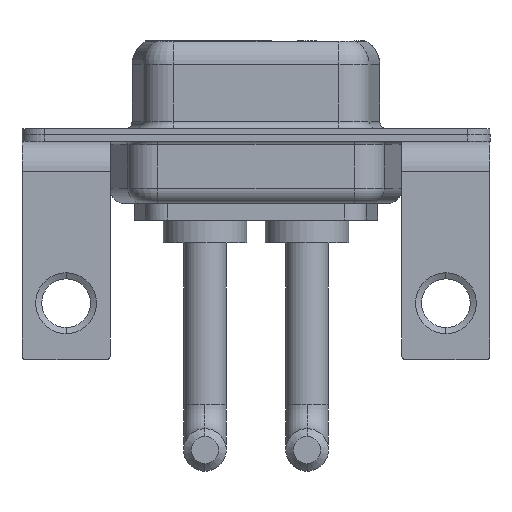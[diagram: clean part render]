
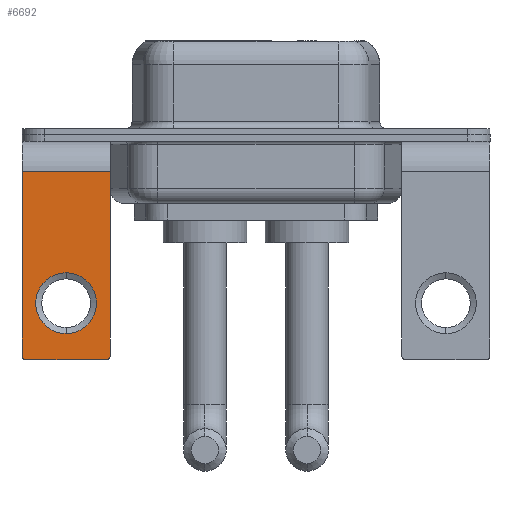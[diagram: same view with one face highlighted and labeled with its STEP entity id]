
A CAD part, front view. The second image highlights one B-rep face of the part: STEP entity #6692.
In plain terms, the highlighted planar face has unit normal (0, -1, 0).
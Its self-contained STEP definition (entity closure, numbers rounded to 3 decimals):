
#91 = ORIENTED_EDGE ( 'NONE', *, *, #12338, .T. ) ;
#143 = VECTOR ( 'NONE', #5828, 1000. ) ;
#197 = VERTEX_POINT ( 'NONE', #11069 ) ;
#400 = VERTEX_POINT ( 'NONE', #3944 ) ;
#421 = LINE ( 'NONE', #5898, #143 ) ;
#467 = ORIENTED_EDGE ( 'NONE', *, *, #11691, .T. ) ;
#588 = VERTEX_POINT ( 'NONE', #7927 ) ;
#1121 = DIRECTION ( 'NONE',  ( -1., 0., 0. ) ) ;
#1144 = CARTESIAN_POINT ( 'NONE',  ( -2.9, -6.25, -2.4 ) ) ;
#1934 = ORIENTED_EDGE ( 'NONE', *, *, #6050, .T. ) ;
#2251 = VERTEX_POINT ( 'NONE', #13970 ) ;
#2392 = VERTEX_POINT ( 'NONE', #5041 ) ;
#2438 = AXIS2_PLACEMENT_3D ( 'NONE', #3745, #2540, #13441 ) ;
#2540 = DIRECTION ( 'NONE',  ( 0., -1., 0. ) ) ;
#2604 = DIRECTION ( 'NONE',  ( 0., 1., 0. ) ) ;
#2614 = EDGE_CURVE ( 'NONE', #13793, #4934, #7477, .T. ) ;
#3727 = EDGE_CURVE ( 'NONE', #2251, #197, #421, .T. ) ;
#3745 = CARTESIAN_POINT ( 'NONE',  ( 2.65, -6.25, -14.55 ) ) ;
#3917 = DIRECTION ( 'NONE',  ( 0., 0., 1. ) ) ;
#3944 = CARTESIAN_POINT ( 'NONE',  ( 0., -6.25, -13.07 ) ) ;
#4039 = CIRCLE ( 'NONE', #14055, 0.25 ) ;
#4110 = EDGE_CURVE ( 'NONE', #2251, #9791, #12003, .T. ) ;
#4293 = AXIS2_PLACEMENT_3D ( 'NONE', #6958, #2604, #12376 ) ;
#4469 = CARTESIAN_POINT ( 'NONE',  ( -2.65, -6.25, -14.55 ) ) ;
#4574 = CARTESIAN_POINT ( 'NONE',  ( 0., -6.25, -11.07 ) ) ;
#4917 = CARTESIAN_POINT ( 'NONE',  ( 0., -6.25, -11.07 ) ) ;
#4934 = VERTEX_POINT ( 'NONE', #7875 ) ;
#4982 = EDGE_CURVE ( 'NONE', #13793, #9791, #10867, .T. ) ;
#5041 = CARTESIAN_POINT ( 'NONE',  ( 0., -6.25, -9.07 ) ) ;
#5447 = CARTESIAN_POINT ( 'NONE',  ( 2.9, -6.25, -2.4 ) ) ;
#5828 = DIRECTION ( 'NONE',  ( -1., 0., 0. ) ) ;
#5898 = CARTESIAN_POINT ( 'NONE',  ( 2.9, -6.25, -14.8 ) ) ;
#5990 = AXIS2_PLACEMENT_3D ( 'NONE', #4917, #8135, #3917 ) ;
#6050 = EDGE_CURVE ( 'NONE', #588, #197, #4039, .T. ) ;
#6692 = ADVANCED_FACE ( 'NONE', ( #13582, #7101 ), #12605, .F. ) ;
#6918 = ORIENTED_EDGE ( 'NONE', *, *, #4982, .F. ) ;
#6957 = ORIENTED_EDGE ( 'NONE', *, *, #2614, .T. ) ;
#6958 = CARTESIAN_POINT ( 'NONE',  ( 2.9, -6.25, -2.4 ) ) ;
#6978 = ORIENTED_EDGE ( 'NONE', *, *, #12125, .T. ) ;
#7101 = FACE_OUTER_BOUND ( 'NONE', #11207, .T. ) ;
#7348 = CARTESIAN_POINT ( 'NONE',  ( 2.9, -6.25, -14.55 ) ) ;
#7477 = LINE ( 'NONE', #11751, #14015 ) ;
#7875 = CARTESIAN_POINT ( 'NONE',  ( -2.9, -6.25, -2.4 ) ) ;
#7899 = DIRECTION ( 'NONE',  ( 0., 0., 1. ) ) ;
#7927 = CARTESIAN_POINT ( 'NONE',  ( -2.9, -6.25, -14.55 ) ) ;
#8135 = DIRECTION ( 'NONE',  ( 0., 1., 0. ) ) ;
#8447 = ORIENTED_EDGE ( 'NONE', *, *, #4110, .T. ) ;
#8491 = VECTOR ( 'NONE', #9982, 1000. ) ;
#8582 = VECTOR ( 'NONE', #10932, 1000. ) ;
#9791 = VERTEX_POINT ( 'NONE', #7348 ) ;
#9853 = DIRECTION ( 'NONE',  ( 0., 0., 1. ) ) ;
#9982 = DIRECTION ( 'NONE',  ( 0., 0., -1. ) ) ;
#10298 = CIRCLE ( 'NONE', #10754, 2. ) ;
#10491 = EDGE_LOOP ( 'NONE', ( #467, #91 ) ) ;
#10752 = ORIENTED_EDGE ( 'NONE', *, *, #3727, .F. ) ;
#10754 = AXIS2_PLACEMENT_3D ( 'NONE', #4574, #12070, #9853 ) ;
#10867 = LINE ( 'NONE', #5447, #8582 ) ;
#10906 = LINE ( 'NONE', #1144, #8491 ) ;
#10932 = DIRECTION ( 'NONE',  ( 0., 0., -1. ) ) ;
#11069 = CARTESIAN_POINT ( 'NONE',  ( -2.65, -6.25, -14.8 ) ) ;
#11207 = EDGE_LOOP ( 'NONE', ( #6978, #1934, #10752, #8447, #6918, #6957 ) ) ;
#11691 = EDGE_CURVE ( 'NONE', #400, #2392, #10298, .T. ) ;
#11751 = CARTESIAN_POINT ( 'NONE',  ( 2.9, -6.25, -2.4 ) ) ;
#11913 = CARTESIAN_POINT ( 'NONE',  ( 2.9, -6.25, -2.4 ) ) ;
#12003 = CIRCLE ( 'NONE', #2438, 0.25 ) ;
#12070 = DIRECTION ( 'NONE',  ( 0., 1., 0. ) ) ;
#12125 = EDGE_CURVE ( 'NONE', #4934, #588, #10906, .T. ) ;
#12338 = EDGE_CURVE ( 'NONE', #2392, #400, #13266, .T. ) ;
#12376 = DIRECTION ( 'NONE',  ( 0., 0., 1. ) ) ;
#12605 = PLANE ( 'NONE',  #4293 ) ;
#13164 = DIRECTION ( 'NONE',  ( 0., -1., 0. ) ) ;
#13266 = CIRCLE ( 'NONE', #5990, 2. ) ;
#13441 = DIRECTION ( 'NONE',  ( 0., 0., 1. ) ) ;
#13582 = FACE_BOUND ( 'NONE', #10491, .T. ) ;
#13793 = VERTEX_POINT ( 'NONE', #11913 ) ;
#13970 = CARTESIAN_POINT ( 'NONE',  ( 2.65, -6.25, -14.8 ) ) ;
#14015 = VECTOR ( 'NONE', #1121, 1000. ) ;
#14055 = AXIS2_PLACEMENT_3D ( 'NONE', #4469, #13164, #7899 ) ;
